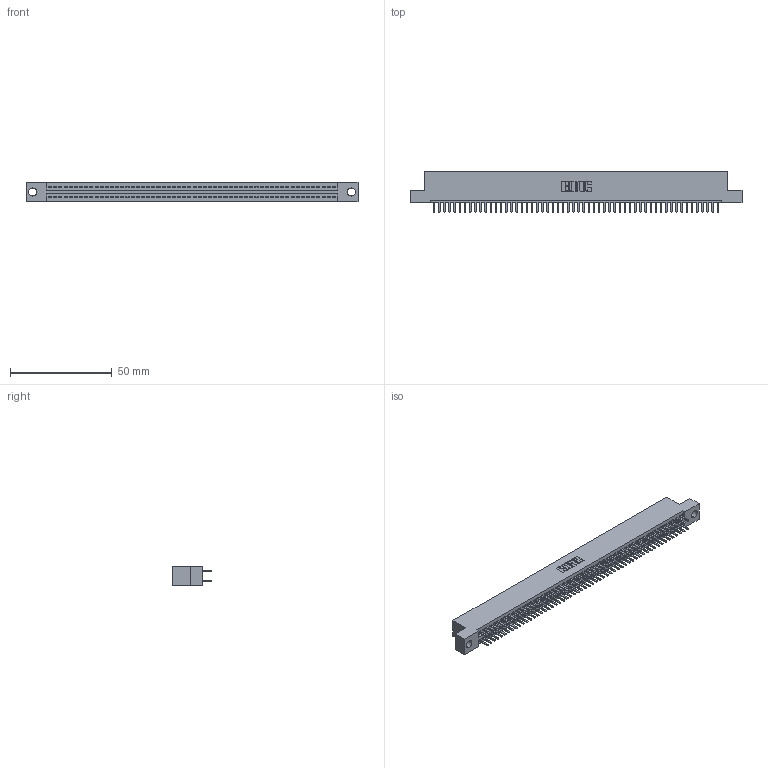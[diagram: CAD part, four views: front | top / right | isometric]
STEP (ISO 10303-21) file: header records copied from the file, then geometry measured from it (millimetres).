
FILE_DESCRIPTION (( 'STEP AP203' ), '1' );
FILE_NAME ('395-112-520-204.STEP', '2021-06-17T18:02:57', ( '' ), ( '' ), 'SwSTEP 2.0', 'SolidWorks 2020', '' );
FILE_SCHEMA (( 'CONFIG_CONTROL_DESIGN' ));
Length unit declared in the file: inch
Products named in the file (3): 345-292-001_345-293-120; 395-112-520-204; 345 Part_Flush Mounting Lugs - 0.156 Dia-TI
Assembly tree (113 placements, depth 2):
  395-112-520-204
    345 Part_Flush Mounting Lugs - 0.156 Dia-TI
    345-292-001_345-293-120  x112
Bounding box: 163.45 x 19.68 x 9.4 mm (x, y, z)
Volume: 15852.4 mm3; surface area: 23450.5 mm2
Topology: 113 solids, 113 shells, 6188 faces, 17961 edges, 11674 vertices
Faces by surface type: plane 4014, cylinder 2174
Entity records: 42587 total; most frequent: CARTESIAN_POINT 7142, ORIENTED_EDGE 7062, DIRECTION 6267, EDGE_CURVE 3531, LINE 3171, VECTOR 3171, VERTEX_POINT 2350, AXIS2_PLACEMENT_3D 1548
